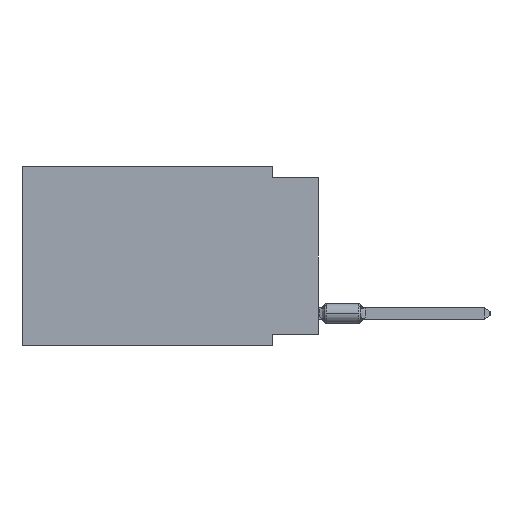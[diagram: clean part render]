
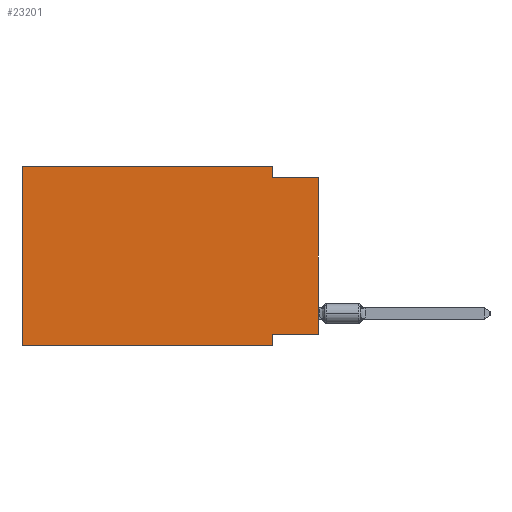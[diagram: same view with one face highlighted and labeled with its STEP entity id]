
A CAD part, left-side view. The second image highlights one B-rep face of the part: STEP entity #23201.
In plain terms, the highlighted planar face has unit normal (-1, 0, 0).
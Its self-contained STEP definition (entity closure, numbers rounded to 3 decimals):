
#727 = DIRECTION ( 'NONE',  ( 0., -1., 0. ) ) ;
#1005 = EDGE_CURVE ( 'NONE', #26022, #18142, #14596, .T. ) ;
#1099 = VECTOR ( 'NONE', #7042, 1000. ) ;
#1172 = VECTOR ( 'NONE', #2000, 1000. ) ;
#2000 = DIRECTION ( 'NONE',  ( 0., 0., 1. ) ) ;
#2302 = ORIENTED_EDGE ( 'NONE', *, *, #14990, .F. ) ;
#2779 = DIRECTION ( 'NONE',  ( 0., 0., -1. ) ) ;
#3254 = CARTESIAN_POINT ( 'NONE',  ( 0., 16.383, 0. ) ) ;
#4590 = VERTEX_POINT ( 'NONE', #6988 ) ;
#4955 = CARTESIAN_POINT ( 'NONE',  ( 0., 2.54, -9.271 ) ) ;
#6959 = VECTOR ( 'NONE', #10639, 1000. ) ;
#6988 = CARTESIAN_POINT ( 'NONE',  ( 0., 2.54, -9.906 ) ) ;
#7042 = DIRECTION ( 'NONE',  ( 0., 0., 1. ) ) ;
#9505 = VERTEX_POINT ( 'NONE', #41042 ) ;
#10639 = DIRECTION ( 'NONE',  ( 0., 1., 0. ) ) ;
#11449 = LINE ( 'NONE', #40590, #1099 ) ;
#11573 = ORIENTED_EDGE ( 'NONE', *, *, #46482, .F. ) ;
#13538 = ORIENTED_EDGE ( 'NONE', *, *, #16152, .T. ) ;
#14596 = LINE ( 'NONE', #34130, #24827 ) ;
#14990 = EDGE_CURVE ( 'NONE', #43509, #15483, #11449, .T. ) ;
#15483 = VERTEX_POINT ( 'NONE', #23369 ) ;
#15559 = DIRECTION ( 'NONE',  ( 0., -1., 0. ) ) ;
#15792 = VECTOR ( 'NONE', #40888, 1000. ) ;
#15981 = CARTESIAN_POINT ( 'NONE',  ( 0., 2.54, -0.635 ) ) ;
#16152 = EDGE_CURVE ( 'NONE', #47378, #18142, #46309, .T. ) ;
#17543 = CARTESIAN_POINT ( 'NONE',  ( 0., 0., -9.271 ) ) ;
#17834 = ORIENTED_EDGE ( 'NONE', *, *, #30143, .F. ) ;
#18142 = VERTEX_POINT ( 'NONE', #36312 ) ;
#18184 = EDGE_CURVE ( 'NONE', #9505, #26022, #25540, .T. ) ;
#20979 = VECTOR ( 'NONE', #45012, 1000. ) ;
#21880 = DIRECTION ( 'NONE',  ( 0., 0., -1. ) ) ;
#23010 = CARTESIAN_POINT ( 'NONE',  ( 0., 16.383, -9.906 ) ) ;
#23018 = LINE ( 'NONE', #37933, #29924 ) ;
#23201 = ADVANCED_FACE ( 'NONE', ( #40213 ), #25520, .F. ) ;
#23369 = CARTESIAN_POINT ( 'NONE',  ( 0., 16.383, 0. ) ) ;
#23774 = CARTESIAN_POINT ( 'NONE',  ( 0., 16.383, -9.906 ) ) ;
#24827 = VECTOR ( 'NONE', #15559, 1000. ) ;
#25520 = PLANE ( 'NONE',  #36868 ) ;
#25540 = LINE ( 'NONE', #45109, #45848 ) ;
#26022 = VERTEX_POINT ( 'NONE', #15981 ) ;
#26897 = EDGE_LOOP ( 'NONE', ( #13538, #35380, #44039, #11573, #2302, #44775, #17834, #31041 ) ) ;
#27387 = CARTESIAN_POINT ( 'NONE',  ( 0., 0., -9.271 ) ) ;
#29924 = VECTOR ( 'NONE', #727, 1000. ) ;
#30143 = EDGE_CURVE ( 'NONE', #39830, #4590, #48191, .T. ) ;
#31041 = ORIENTED_EDGE ( 'NONE', *, *, #31564, .F. ) ;
#31564 = EDGE_CURVE ( 'NONE', #47378, #39830, #47859, .T. ) ;
#32345 = CARTESIAN_POINT ( 'NONE',  ( 0., 0., 0. ) ) ;
#34130 = CARTESIAN_POINT ( 'NONE',  ( 0., 0., -0.635 ) ) ;
#35380 = ORIENTED_EDGE ( 'NONE', *, *, #1005, .F. ) ;
#36312 = CARTESIAN_POINT ( 'NONE',  ( 0., 0., -0.635 ) ) ;
#36868 = AXIS2_PLACEMENT_3D ( 'NONE', #3254, #40447, #2779 ) ;
#37933 = CARTESIAN_POINT ( 'NONE',  ( 0., 16.383, 0. ) ) ;
#39830 = VERTEX_POINT ( 'NONE', #4955 ) ;
#40213 = FACE_OUTER_BOUND ( 'NONE', #26897, .T. ) ;
#40447 = DIRECTION ( 'NONE',  ( 1., 0., 0. ) ) ;
#40590 = CARTESIAN_POINT ( 'NONE',  ( 0., 16.383, 0. ) ) ;
#40888 = DIRECTION ( 'NONE',  ( 0., -1., 0. ) ) ;
#41042 = CARTESIAN_POINT ( 'NONE',  ( 0., 2.54, 0. ) ) ;
#41340 = CARTESIAN_POINT ( 'NONE',  ( 0., 2.54, -9.906 ) ) ;
#43509 = VERTEX_POINT ( 'NONE', #23774 ) ;
#44039 = ORIENTED_EDGE ( 'NONE', *, *, #18184, .F. ) ;
#44775 = ORIENTED_EDGE ( 'NONE', *, *, #47216, .T. ) ;
#45012 = DIRECTION ( 'NONE',  ( 0., 0., -1. ) ) ;
#45032 = LINE ( 'NONE', #23010, #15792 ) ;
#45109 = CARTESIAN_POINT ( 'NONE',  ( 0., 2.54, 0. ) ) ;
#45848 = VECTOR ( 'NONE', #21880, 1000. ) ;
#46309 = LINE ( 'NONE', #32345, #1172 ) ;
#46482 = EDGE_CURVE ( 'NONE', #15483, #9505, #23018, .T. ) ;
#47216 = EDGE_CURVE ( 'NONE', #43509, #4590, #45032, .T. ) ;
#47378 = VERTEX_POINT ( 'NONE', #27387 ) ;
#47859 = LINE ( 'NONE', #17543, #6959 ) ;
#48191 = LINE ( 'NONE', #41340, #20979 ) ;
